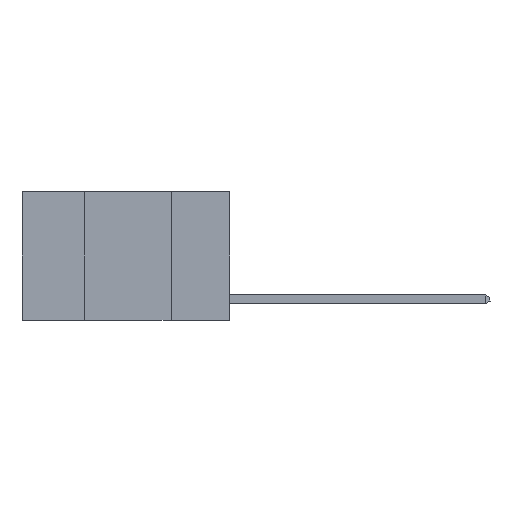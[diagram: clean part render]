
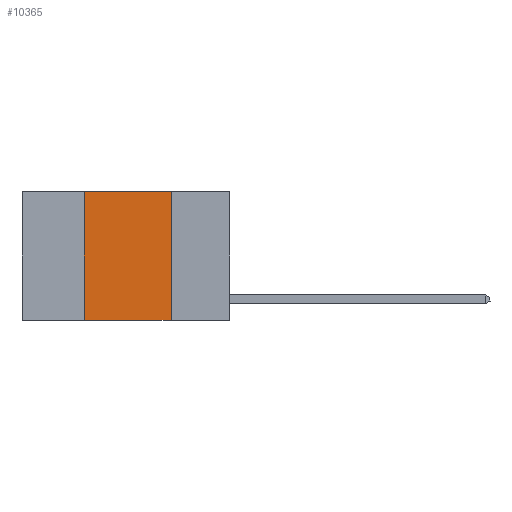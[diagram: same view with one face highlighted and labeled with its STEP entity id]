
A CAD part, left-side view. The second image highlights one B-rep face of the part: STEP entity #10365.
In plain terms, the highlighted planar face has unit normal (-1, 0, 0).
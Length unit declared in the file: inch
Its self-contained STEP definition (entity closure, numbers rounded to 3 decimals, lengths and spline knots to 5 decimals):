
#1223 = LINE ( 'NONE', #9113, #25375 ) ;
#1480 = DIRECTION ( 'NONE',  ( 0., 0., 1. ) ) ;
#4850 = VERTEX_POINT ( 'NONE', #21149 ) ;
#5812 = VERTEX_POINT ( 'NONE', #22410 ) ;
#6062 = LINE ( 'NONE', #29598, #17653 ) ;
#6623 = FACE_OUTER_BOUND ( 'NONE', #18598, .T. ) ;
#6966 = AXIS2_PLACEMENT_3D ( 'NONE', #24840, #10853, #27181 ) ;
#7931 = ORIENTED_EDGE ( 'NONE', *, *, #19047, .F. ) ;
#8543 = PLANE ( 'NONE',  #6966 ) ;
#9113 = CARTESIAN_POINT ( 'NONE',  ( 0., 0.6, -0.37 ) ) ;
#10365 = ADVANCED_FACE ( 'NONE', ( #6623 ), #8543, .F. ) ;
#10485 = VERTEX_POINT ( 'NONE', #25350 ) ;
#10853 = DIRECTION ( 'NONE',  ( 1., 0., 0. ) ) ;
#11295 = LINE ( 'NONE', #13332, #16015 ) ;
#13161 = CARTESIAN_POINT ( 'NONE',  ( 0., 0.42, 0. ) ) ;
#13332 = CARTESIAN_POINT ( 'NONE',  ( 0., 0.17, 0. ) ) ;
#13349 = EDGE_CURVE ( 'NONE', #10485, #4850, #11295, .T. ) ;
#13670 = LINE ( 'NONE', #13161, #19131 ) ;
#15551 = ORIENTED_EDGE ( 'NONE', *, *, #27428, .T. ) ;
#16015 = VECTOR ( 'NONE', #18007, 39.37008 ) ;
#17653 = VECTOR ( 'NONE', #25003, 39.37008 ) ;
#18007 = DIRECTION ( 'NONE',  ( 0., 0., -1. ) ) ;
#18598 = EDGE_LOOP ( 'NONE', ( #19568, #7931, #27245, #15551 ) ) ;
#19006 = EDGE_CURVE ( 'NONE', #5812, #21708, #13670, .T. ) ;
#19047 = EDGE_CURVE ( 'NONE', #21708, #10485, #6062, .T. ) ;
#19131 = VECTOR ( 'NONE', #1480, 39.37008 ) ;
#19568 = ORIENTED_EDGE ( 'NONE', *, *, #13349, .F. ) ;
#21149 = CARTESIAN_POINT ( 'NONE',  ( 0., 0.17, -0.37 ) ) ;
#21708 = VERTEX_POINT ( 'NONE', #25738 ) ;
#22410 = CARTESIAN_POINT ( 'NONE',  ( 0., 0.42, -0.37 ) ) ;
#24840 = CARTESIAN_POINT ( 'NONE',  ( 0., 0.6, 0. ) ) ;
#25003 = DIRECTION ( 'NONE',  ( 0., -1., 0. ) ) ;
#25350 = CARTESIAN_POINT ( 'NONE',  ( 0., 0.17, 0. ) ) ;
#25375 = VECTOR ( 'NONE', #30127, 39.37008 ) ;
#25738 = CARTESIAN_POINT ( 'NONE',  ( 0., 0.42, 0. ) ) ;
#27181 = DIRECTION ( 'NONE',  ( 0., 0., -1. ) ) ;
#27245 = ORIENTED_EDGE ( 'NONE', *, *, #19006, .F. ) ;
#27428 = EDGE_CURVE ( 'NONE', #5812, #4850, #1223, .T. ) ;
#29598 = CARTESIAN_POINT ( 'NONE',  ( 0., 0.6, 0. ) ) ;
#30127 = DIRECTION ( 'NONE',  ( 0., -1., 0. ) ) ;
